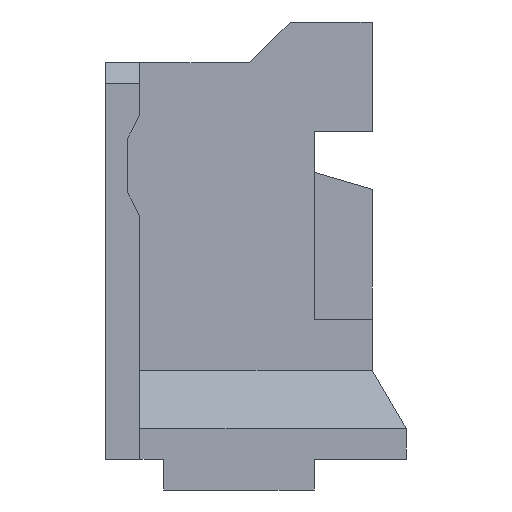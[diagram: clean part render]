
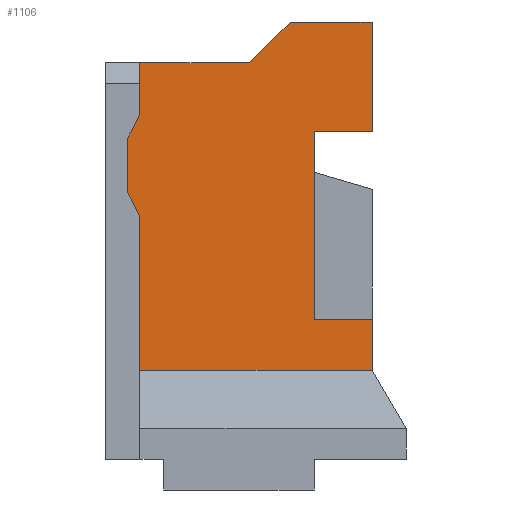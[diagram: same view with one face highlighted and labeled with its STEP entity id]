
A CAD part, left-side view. The second image highlights one B-rep face of the part: STEP entity #1106.
In plain terms, the highlighted planar face has unit normal (-1, 0, 0).
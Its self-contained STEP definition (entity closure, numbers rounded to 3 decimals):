
#408 = CARTESIAN_POINT ( 'NONE',  ( -1.25, 1.1, 0. ) ) ;
#455 = ORIENTED_EDGE ( 'NONE', *, *, #9222, .F. ) ;
#495 = CARTESIAN_POINT ( 'NONE',  ( -1.25, 1.275, -1.9 ) ) ;
#547 = LINE ( 'NONE', #5971, #9213 ) ;
#623 = ORIENTED_EDGE ( 'NONE', *, *, #8844, .F. ) ;
#665 = EDGE_CURVE ( 'NONE', #10793, #882, #12798, .T. ) ;
#755 = CARTESIAN_POINT ( 'NONE',  ( -1.25, 1.1, -5.8 ) ) ;
#882 = VERTEX_POINT ( 'NONE', #11633 ) ;
#1098 = EDGE_CURVE ( 'NONE', #10182, #5012, #5931, .T. ) ;
#1106 = ADVANCED_FACE ( 'NONE', ( #9152 ), #2473, .F. ) ;
#1364 = LINE ( 'NONE', #11672, #3513 ) ;
#1443 = DIRECTION ( 'NONE',  ( 0., 0., 1. ) ) ;
#1449 = CARTESIAN_POINT ( 'NONE',  ( -1.25, 0., 0. ) ) ;
#1530 = CARTESIAN_POINT ( 'NONE',  ( -1.25, -3., -4.5 ) ) ;
#1787 = VECTOR ( 'NONE', #13041, 1000. ) ;
#1798 = CARTESIAN_POINT ( 'NONE',  ( -1.25, 1.1, -4.5 ) ) ;
#1819 = CARTESIAN_POINT ( 'NONE',  ( -1.25, 3.057, -3.75 ) ) ;
#1966 = EDGE_CURVE ( 'NONE', #13379, #10818, #11184, .T. ) ;
#2395 = DIRECTION ( 'NONE',  ( 0., 0., 1. ) ) ;
#2473 = PLANE ( 'NONE',  #8905 ) ;
#2612 = LINE ( 'NONE', #1819, #9938 ) ;
#2648 = DIRECTION ( 'NONE',  ( 0., 1., 0. ) ) ;
#2797 = CARTESIAN_POINT ( 'NONE',  ( -1.25, -2.3, -1. ) ) ;
#2899 = ORIENTED_EDGE ( 'NONE', *, *, #1098, .F. ) ;
#3167 = ORIENTED_EDGE ( 'NONE', *, *, #7894, .F. ) ;
#3513 = VECTOR ( 'NONE', #7511, 1000. ) ;
#3679 = VERTEX_POINT ( 'NONE', #9553 ) ;
#3716 = DIRECTION ( 'NONE',  ( 0., 1., 0. ) ) ;
#3797 = VECTOR ( 'NONE', #3716, 1000. ) ;
#3897 = VERTEX_POINT ( 'NONE', #408 ) ;
#3908 = DIRECTION ( 'NONE',  ( 0., -0.447, 0.894 ) ) ;
#4006 = VERTEX_POINT ( 'NONE', #495 ) ;
#4044 = DIRECTION ( 'NONE',  ( 0., -1., 0. ) ) ;
#4128 = EDGE_CURVE ( 'NONE', #3897, #3679, #12626, .T. ) ;
#4240 = CARTESIAN_POINT ( 'NONE',  ( -1.25, -1.1, 0.6 ) ) ;
#4418 = LINE ( 'NONE', #7720, #7969 ) ;
#4555 = EDGE_CURVE ( 'NONE', #8438, #4006, #9812, .T. ) ;
#4588 = CARTESIAN_POINT ( 'NONE',  ( -1.25, -1.45, -3.75 ) ) ;
#4628 = VECTOR ( 'NONE', #5508, 1000. ) ;
#4762 = CARTESIAN_POINT ( 'NONE',  ( -1.25, 1.275, -1.1 ) ) ;
#5012 = VERTEX_POINT ( 'NONE', #9451 ) ;
#5091 = EDGE_CURVE ( 'NONE', #4006, #6690, #4418, .T. ) ;
#5365 = ORIENTED_EDGE ( 'NONE', *, *, #5091, .F. ) ;
#5463 = CARTESIAN_POINT ( 'NONE',  ( -1.25, 1.1, -0.75 ) ) ;
#5508 = DIRECTION ( 'NONE',  ( 0., 0., -1. ) ) ;
#5608 = CARTESIAN_POINT ( 'NONE',  ( -1.25, 1.1, -2.25 ) ) ;
#5769 = LINE ( 'NONE', #1530, #8329 ) ;
#5781 = LINE ( 'NONE', #11368, #9002 ) ;
#5823 = ORIENTED_EDGE ( 'NONE', *, *, #9252, .F. ) ;
#5931 = LINE ( 'NONE', #10619, #4628 ) ;
#5971 = CARTESIAN_POINT ( 'NONE',  ( -1.25, -2.3, 0.6 ) ) ;
#6079 = LINE ( 'NONE', #11149, #12111 ) ;
#6187 = DIRECTION ( 'NONE',  ( 0., -0.707, 0.707 ) ) ;
#6205 = ORIENTED_EDGE ( 'NONE', *, *, #10410, .F. ) ;
#6412 = ORIENTED_EDGE ( 'NONE', *, *, #7406, .F. ) ;
#6640 = VERTEX_POINT ( 'NONE', #4588 ) ;
#6690 = VERTEX_POINT ( 'NONE', #4762 ) ;
#7189 = VECTOR ( 'NONE', #4044, 1000. ) ;
#7406 = EDGE_CURVE ( 'NONE', #10818, #10793, #547, .T. ) ;
#7511 = DIRECTION ( 'NONE',  ( 0., 0., -1. ) ) ;
#7659 = DIRECTION ( 'NONE',  ( 0., 0., -1. ) ) ;
#7720 = CARTESIAN_POINT ( 'NONE',  ( -1.25, 1.275, -2.25 ) ) ;
#7894 = EDGE_CURVE ( 'NONE', #882, #6640, #1364, .T. ) ;
#7969 = VECTOR ( 'NONE', #2395, 1000. ) ;
#8169 = CARTESIAN_POINT ( 'NONE',  ( -1.25, 1.1, 0. ) ) ;
#8329 = VECTOR ( 'NONE', #2648, 1000. ) ;
#8438 = VERTEX_POINT ( 'NONE', #13433 ) ;
#8501 = CARTESIAN_POINT ( 'NONE',  ( -1.25, -1.1, 0.6 ) ) ;
#8595 = CARTESIAN_POINT ( 'NONE',  ( -1.25, -2.3, -1. ) ) ;
#8633 = DIRECTION ( 'NONE',  ( 0., -1., 0. ) ) ;
#8733 = VECTOR ( 'NONE', #8633, 1000. ) ;
#8844 = EDGE_CURVE ( 'NONE', #3679, #13379, #5781, .T. ) ;
#8905 = AXIS2_PLACEMENT_3D ( 'NONE', #1449, #11776, #7659 ) ;
#9002 = VECTOR ( 'NONE', #6187, 1000. ) ;
#9152 = FACE_OUTER_BOUND ( 'NONE', #9736, .T. ) ;
#9213 = VECTOR ( 'NONE', #12177, 1000. ) ;
#9222 = EDGE_CURVE ( 'NONE', #5012, #9454, #5769, .T. ) ;
#9252 = EDGE_CURVE ( 'NONE', #9454, #8438, #9312, .T. ) ;
#9312 = LINE ( 'NONE', #9761, #12791 ) ;
#9451 = CARTESIAN_POINT ( 'NONE',  ( -1.25, -2.3, -4.5 ) ) ;
#9454 = VERTEX_POINT ( 'NONE', #1798 ) ;
#9553 = CARTESIAN_POINT ( 'NONE',  ( -1.25, -0.5, 0. ) ) ;
#9586 = EDGE_CURVE ( 'NONE', #6690, #10638, #6079, .T. ) ;
#9736 = EDGE_LOOP ( 'NONE', ( #6205, #9757, #5365, #13406, #5823, #455, #2899, #10311, #3167, #11093, #6412, #13266, #623, #12167 ) ) ;
#9757 = ORIENTED_EDGE ( 'NONE', *, *, #9586, .F. ) ;
#9761 = CARTESIAN_POINT ( 'NONE',  ( -1.25, 1.1, -5.8 ) ) ;
#9812 = LINE ( 'NONE', #5608, #1787 ) ;
#9938 = VECTOR ( 'NONE', #13274, 1000. ) ;
#10163 = CARTESIAN_POINT ( 'NONE',  ( -1.25, -2.3, -3.75 ) ) ;
#10182 = VERTEX_POINT ( 'NONE', #10163 ) ;
#10311 = ORIENTED_EDGE ( 'NONE', *, *, #10329, .F. ) ;
#10329 = EDGE_CURVE ( 'NONE', #6640, #10182, #2612, .T. ) ;
#10410 = EDGE_CURVE ( 'NONE', #10638, #3897, #10746, .T. ) ;
#10588 = VECTOR ( 'NONE', #11183, 1000. ) ;
#10619 = CARTESIAN_POINT ( 'NONE',  ( -1.25, -2.3, -1.85 ) ) ;
#10638 = VERTEX_POINT ( 'NONE', #5463 ) ;
#10746 = LINE ( 'NONE', #755, #10588 ) ;
#10793 = VERTEX_POINT ( 'NONE', #8595 ) ;
#10818 = VERTEX_POINT ( 'NONE', #12886 ) ;
#11093 = ORIENTED_EDGE ( 'NONE', *, *, #665, .F. ) ;
#11149 = CARTESIAN_POINT ( 'NONE',  ( -1.25, 1.1, -0.75 ) ) ;
#11183 = DIRECTION ( 'NONE',  ( 0., 0., 1. ) ) ;
#11184 = LINE ( 'NONE', #8501, #8733 ) ;
#11368 = CARTESIAN_POINT ( 'NONE',  ( -1.25, -0.5, 0. ) ) ;
#11633 = CARTESIAN_POINT ( 'NONE',  ( -1.25, -1.45, -1. ) ) ;
#11672 = CARTESIAN_POINT ( 'NONE',  ( -1.25, -1.45, -1. ) ) ;
#11776 = DIRECTION ( 'NONE',  ( 1., 0., 0. ) ) ;
#12111 = VECTOR ( 'NONE', #3908, 1000. ) ;
#12167 = ORIENTED_EDGE ( 'NONE', *, *, #4128, .F. ) ;
#12177 = DIRECTION ( 'NONE',  ( 0., 0., -1. ) ) ;
#12626 = LINE ( 'NONE', #8169, #7189 ) ;
#12791 = VECTOR ( 'NONE', #1443, 1000. ) ;
#12798 = LINE ( 'NONE', #2797, #3797 ) ;
#12886 = CARTESIAN_POINT ( 'NONE',  ( -1.25, -2.3, 0.6 ) ) ;
#13041 = DIRECTION ( 'NONE',  ( 0., 0.447, 0.894 ) ) ;
#13266 = ORIENTED_EDGE ( 'NONE', *, *, #1966, .F. ) ;
#13274 = DIRECTION ( 'NONE',  ( 0., -1., 0. ) ) ;
#13379 = VERTEX_POINT ( 'NONE', #4240 ) ;
#13406 = ORIENTED_EDGE ( 'NONE', *, *, #4555, .F. ) ;
#13433 = CARTESIAN_POINT ( 'NONE',  ( -1.25, 1.1, -2.25 ) ) ;
